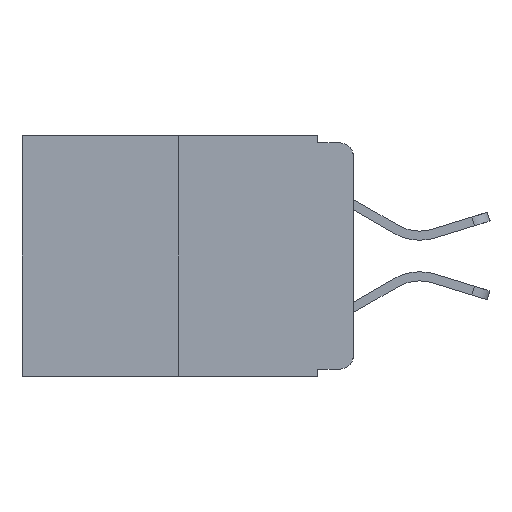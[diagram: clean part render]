
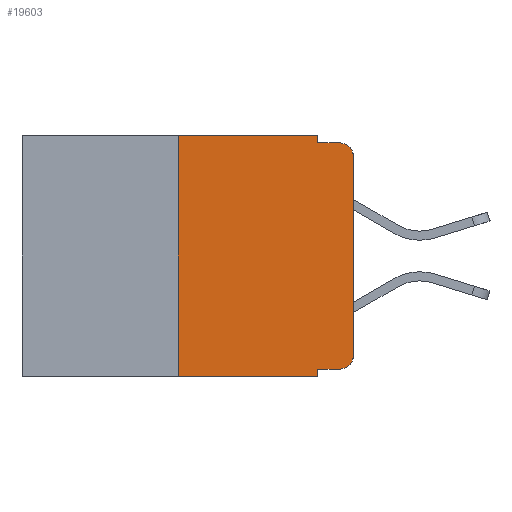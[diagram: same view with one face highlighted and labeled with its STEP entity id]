
A CAD part, left-side view. The second image highlights one B-rep face of the part: STEP entity #19603.
In plain terms, the highlighted planar face has unit normal (-1, 0, 0).
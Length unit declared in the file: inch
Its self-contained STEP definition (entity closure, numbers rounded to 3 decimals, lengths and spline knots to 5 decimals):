
#570 = DIRECTION ( 'NONE',  ( -1., 0., 0. ) ) ;
#1470 = CARTESIAN_POINT ( 'NONE',  ( 0., 0.02, -0.313 ) ) ;
#1594 = CARTESIAN_POINT ( 'NONE',  ( 0., 0.25, 0. ) ) ;
#1757 = DIRECTION ( 'NONE',  ( 0., 0., -1. ) ) ;
#2749 = DIRECTION ( 'NONE',  ( 0., 0., 1. ) ) ;
#3366 = LINE ( 'NONE', #7154, #9933 ) ;
#3835 = VECTOR ( 'NONE', #20340, 39.37008 ) ;
#4148 = VERTEX_POINT ( 'NONE', #1594 ) ;
#4190 = EDGE_CURVE ( 'NONE', #9328, #9346, #16593, .T. ) ;
#4249 = LINE ( 'NONE', #15421, #5931 ) ;
#4306 = CARTESIAN_POINT ( 'NONE',  ( 0., 0.473, 0. ) ) ;
#5496 = VERTEX_POINT ( 'NONE', #11388 ) ;
#5522 = DIRECTION ( 'NONE',  ( 0., 0., -1. ) ) ;
#5931 = VECTOR ( 'NONE', #19307, 39.37008 ) ;
#6033 = CARTESIAN_POINT ( 'NONE',  ( 0., 0., 0. ) ) ;
#6419 = ORIENTED_EDGE ( 'NONE', *, *, #17134, .F. ) ;
#6426 = EDGE_CURVE ( 'NONE', #9346, #10314, #20990, .T. ) ;
#6572 = ORIENTED_EDGE ( 'NONE', *, *, #13170, .F. ) ;
#6624 = DIRECTION ( 'NONE',  ( 0., -1., 0. ) ) ;
#6653 = CARTESIAN_POINT ( 'NONE',  ( 0., 0.051, -0.01 ) ) ;
#6709 = CARTESIAN_POINT ( 'NONE',  ( 0., 0.051, -0.01 ) ) ;
#6728 = VERTEX_POINT ( 'NONE', #22356 ) ;
#7000 = EDGE_CURVE ( 'NONE', #15851, #9328, #10377, .T. ) ;
#7154 = CARTESIAN_POINT ( 'NONE',  ( 0., 0.051, 0. ) ) ;
#7560 = DIRECTION ( 'NONE',  ( 0., -1., 0. ) ) ;
#7754 = CARTESIAN_POINT ( 'NONE',  ( 0., 0.051, 0. ) ) ;
#7769 = ORIENTED_EDGE ( 'NONE', *, *, #11361, .F. ) ;
#8241 = AXIS2_PLACEMENT_3D ( 'NONE', #4306, #15048, #5522 ) ;
#9328 = VERTEX_POINT ( 'NONE', #22031 ) ;
#9346 = VERTEX_POINT ( 'NONE', #22148 ) ;
#9452 = EDGE_LOOP ( 'NONE', ( #11535, #14718, #22354, #20757, #7769, #6572, #12692, #6419, #14800, #22252 ) ) ;
#9473 = VECTOR ( 'NONE', #11550, 39.37008 ) ;
#9924 = EDGE_CURVE ( 'NONE', #10314, #6728, #18404, .T. ) ;
#9933 = VECTOR ( 'NONE', #10887, 39.37008 ) ;
#10033 = CARTESIAN_POINT ( 'NONE',  ( 0., 0.25, 0. ) ) ;
#10314 = VERTEX_POINT ( 'NONE', #14769 ) ;
#10377 = LINE ( 'NONE', #18038, #15515 ) ;
#10887 = DIRECTION ( 'NONE',  ( 0., 0., -1. ) ) ;
#11361 = EDGE_CURVE ( 'NONE', #4148, #12840, #15703, .T. ) ;
#11388 = CARTESIAN_POINT ( 'NONE',  ( 0., 0.051, -0.343 ) ) ;
#11510 = LINE ( 'NONE', #7754, #21004 ) ;
#11535 = ORIENTED_EDGE ( 'NONE', *, *, #6426, .T. ) ;
#11550 = DIRECTION ( 'NONE',  ( 0., 0., 1. ) ) ;
#12692 = ORIENTED_EDGE ( 'NONE', *, *, #20312, .T. ) ;
#12840 = VERTEX_POINT ( 'NONE', #20016 ) ;
#13170 = EDGE_CURVE ( 'NONE', #18601, #4148, #23501, .T. ) ;
#13480 = CARTESIAN_POINT ( 'NONE',  ( 0., 0.051, -0.333 ) ) ;
#13841 = FACE_OUTER_BOUND ( 'NONE', #9452, .T. ) ;
#13912 = CARTESIAN_POINT ( 'NONE',  ( 0., 0.02, -0.03 ) ) ;
#14401 = AXIS2_PLACEMENT_3D ( 'NONE', #13912, #570, #1757 ) ;
#14432 = LINE ( 'NONE', #6653, #3835 ) ;
#14467 = VECTOR ( 'NONE', #2749, 39.37008 ) ;
#14718 = ORIENTED_EDGE ( 'NONE', *, *, #9924, .T. ) ;
#14769 = CARTESIAN_POINT ( 'NONE',  ( 0., 0., -0.03 ) ) ;
#14800 = ORIENTED_EDGE ( 'NONE', *, *, #7000, .T. ) ;
#15048 = DIRECTION ( 'NONE',  ( 1., 0., 0. ) ) ;
#15162 = DIRECTION ( 'NONE',  ( 0., 0., -1. ) ) ;
#15421 = CARTESIAN_POINT ( 'NONE',  ( 0., 0.473, -0.343 ) ) ;
#15515 = VECTOR ( 'NONE', #6624, 39.37008 ) ;
#15703 = LINE ( 'NONE', #23380, #21640 ) ;
#15851 = VERTEX_POINT ( 'NONE', #13480 ) ;
#16593 = CIRCLE ( 'NONE', #23847, 0.02 ) ;
#17134 = EDGE_CURVE ( 'NONE', #15851, #5496, #11510, .T. ) ;
#18038 = CARTESIAN_POINT ( 'NONE',  ( 0., 0.051, -0.333 ) ) ;
#18404 = CIRCLE ( 'NONE', #14401, 0.02 ) ;
#18601 = VERTEX_POINT ( 'NONE', #19428 ) ;
#19009 = VERTEX_POINT ( 'NONE', #6709 ) ;
#19307 = DIRECTION ( 'NONE',  ( 0., -1., 0. ) ) ;
#19428 = CARTESIAN_POINT ( 'NONE',  ( 0., 0.25, -0.343 ) ) ;
#19540 = EDGE_CURVE ( 'NONE', #19009, #6728, #14432, .T. ) ;
#19603 = ADVANCED_FACE ( 'NONE', ( #13841 ), #21519, .F. ) ;
#20016 = CARTESIAN_POINT ( 'NONE',  ( 0., 0.051, 0. ) ) ;
#20189 = EDGE_CURVE ( 'NONE', #12840, #19009, #3366, .T. ) ;
#20312 = EDGE_CURVE ( 'NONE', #18601, #5496, #4249, .T. ) ;
#20340 = DIRECTION ( 'NONE',  ( 0., -1., 0. ) ) ;
#20757 = ORIENTED_EDGE ( 'NONE', *, *, #20189, .F. ) ;
#20990 = LINE ( 'NONE', #6033, #9473 ) ;
#21004 = VECTOR ( 'NONE', #15162, 39.37008 ) ;
#21176 = DIRECTION ( 'NONE',  ( 0., 0., -1. ) ) ;
#21519 = PLANE ( 'NONE',  #8241 ) ;
#21640 = VECTOR ( 'NONE', #7560, 39.37008 ) ;
#22031 = CARTESIAN_POINT ( 'NONE',  ( 0., 0.02, -0.333 ) ) ;
#22148 = CARTESIAN_POINT ( 'NONE',  ( 0., 0., -0.313 ) ) ;
#22252 = ORIENTED_EDGE ( 'NONE', *, *, #4190, .T. ) ;
#22354 = ORIENTED_EDGE ( 'NONE', *, *, #19540, .F. ) ;
#22356 = CARTESIAN_POINT ( 'NONE',  ( 0., 0.02, -0.01 ) ) ;
#22721 = DIRECTION ( 'NONE',  ( -1., 0., 0. ) ) ;
#23380 = CARTESIAN_POINT ( 'NONE',  ( 0., 0.473, 0. ) ) ;
#23501 = LINE ( 'NONE', #10033, #14467 ) ;
#23847 = AXIS2_PLACEMENT_3D ( 'NONE', #1470, #22721, #21176 ) ;
